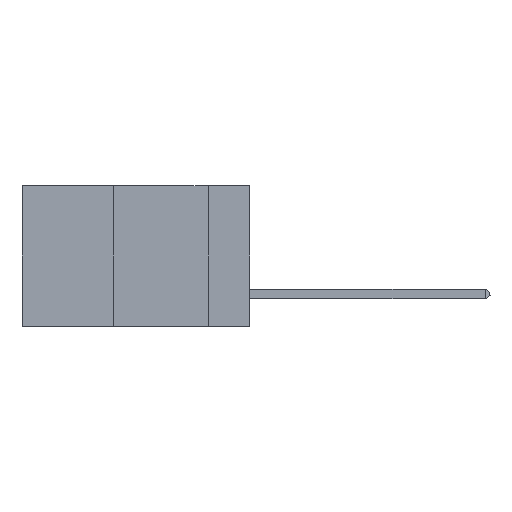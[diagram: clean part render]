
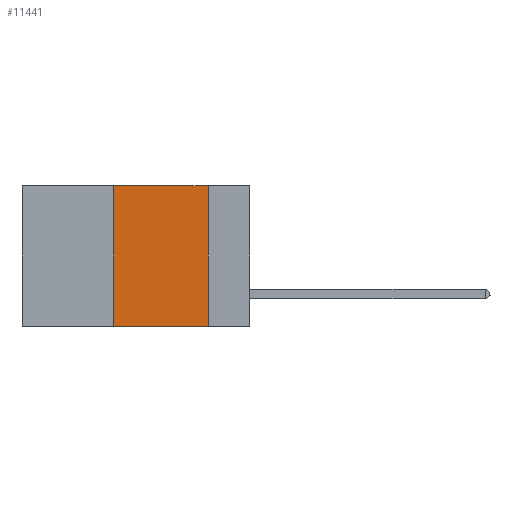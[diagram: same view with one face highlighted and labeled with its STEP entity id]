
A CAD part, left-side view. The second image highlights one B-rep face of the part: STEP entity #11441.
In plain terms, the highlighted planar face has unit normal (-1, 0, 0).
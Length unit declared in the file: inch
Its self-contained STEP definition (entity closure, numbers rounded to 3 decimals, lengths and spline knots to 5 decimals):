
#1 = VERTEX_POINT ( 'NONE', #5794 ) ;
#151 = EDGE_CURVE ( 'NONE', #15165, #3299, #11808, .T. ) ;
#315 = VECTOR ( 'NONE', #11108, 39.37008 ) ;
#334 = EDGE_CURVE ( 'NONE', #1, #15165, #12006, .T. ) ;
#1603 = VERTEX_POINT ( 'NONE', #17304 ) ;
#3299 = VERTEX_POINT ( 'NONE', #12266 ) ;
#4755 = CARTESIAN_POINT ( 'NONE',  ( 0., 0.11, 0. ) ) ;
#4796 = DIRECTION ( 'NONE',  ( 1., 0., 0. ) ) ;
#4802 = FACE_OUTER_BOUND ( 'NONE', #8939, .T. ) ;
#5794 = CARTESIAN_POINT ( 'NONE',  ( 0., 0.36, 0. ) ) ;
#6206 = EDGE_CURVE ( 'NONE', #1603, #1, #7151, .T. ) ;
#7151 = LINE ( 'NONE', #8122, #315 ) ;
#7187 = VECTOR ( 'NONE', #15128, 39.37008 ) ;
#7820 = ORIENTED_EDGE ( 'NONE', *, *, #334, .F. ) ;
#8122 = CARTESIAN_POINT ( 'NONE',  ( 0., 0.36, 0. ) ) ;
#8306 = LINE ( 'NONE', #17421, #17077 ) ;
#8853 = AXIS2_PLACEMENT_3D ( 'NONE', #17523, #4796, #16008 ) ;
#8939 = EDGE_LOOP ( 'NONE', ( #9425, #7820, #15667, #11988 ) ) ;
#9425 = ORIENTED_EDGE ( 'NONE', *, *, #151, .F. ) ;
#10758 = CARTESIAN_POINT ( 'NONE',  ( 0., 0.11, 0. ) ) ;
#11108 = DIRECTION ( 'NONE',  ( 0., 0., 1. ) ) ;
#11441 = ADVANCED_FACE ( 'NONE', ( #4802 ), #11755, .F. ) ;
#11755 = PLANE ( 'NONE',  #8853 ) ;
#11808 = LINE ( 'NONE', #4755, #12902 ) ;
#11988 = ORIENTED_EDGE ( 'NONE', *, *, #14922, .T. ) ;
#12006 = LINE ( 'NONE', #18014, #7187 ) ;
#12266 = CARTESIAN_POINT ( 'NONE',  ( 0., 0.11, -0.37 ) ) ;
#12902 = VECTOR ( 'NONE', #14530, 39.37008 ) ;
#14530 = DIRECTION ( 'NONE',  ( 0., 0., -1. ) ) ;
#14922 = EDGE_CURVE ( 'NONE', #1603, #3299, #8306, .T. ) ;
#15128 = DIRECTION ( 'NONE',  ( 0., -1., 0. ) ) ;
#15165 = VERTEX_POINT ( 'NONE', #10758 ) ;
#15667 = ORIENTED_EDGE ( 'NONE', *, *, #6206, .F. ) ;
#16008 = DIRECTION ( 'NONE',  ( 0., 0., -1. ) ) ;
#16142 = DIRECTION ( 'NONE',  ( 0., -1., 0. ) ) ;
#17077 = VECTOR ( 'NONE', #16142, 39.37008 ) ;
#17304 = CARTESIAN_POINT ( 'NONE',  ( 0., 0.36, -0.37 ) ) ;
#17421 = CARTESIAN_POINT ( 'NONE',  ( 0., 0.6, -0.37 ) ) ;
#17523 = CARTESIAN_POINT ( 'NONE',  ( 0., 0.6, 0. ) ) ;
#18014 = CARTESIAN_POINT ( 'NONE',  ( 0., 0.6, 0. ) ) ;
